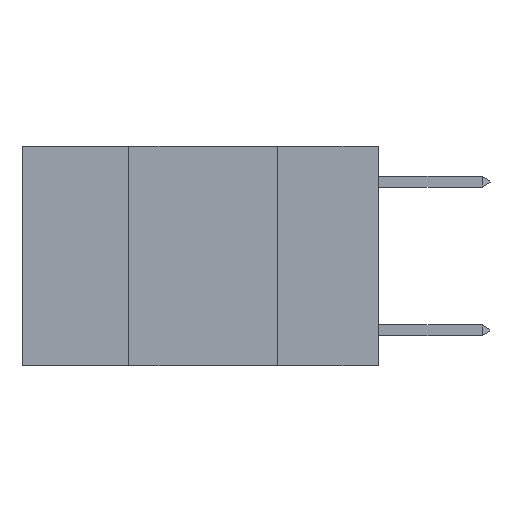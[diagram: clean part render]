
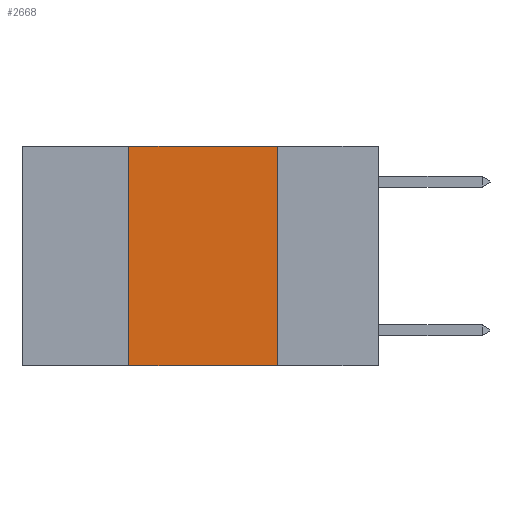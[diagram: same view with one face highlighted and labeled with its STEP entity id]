
A CAD part, left-side view. The second image highlights one B-rep face of the part: STEP entity #2668.
In plain terms, the highlighted planar face has unit normal (-1, 0, 0).
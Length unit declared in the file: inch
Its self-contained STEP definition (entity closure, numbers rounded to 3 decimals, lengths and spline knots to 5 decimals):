
#463 = EDGE_CURVE ( 'NONE', #13449, #3422, #1289, .T. ) ;
#912 = FACE_OUTER_BOUND ( 'NONE', #4843, .T. ) ;
#996 = DIRECTION ( 'NONE',  ( 0., 0., -1. ) ) ;
#1289 = LINE ( 'NONE', #12837, #10426 ) ;
#1579 = LINE ( 'NONE', #11140, #13060 ) ;
#1795 = EDGE_CURVE ( 'NONE', #3422, #13500, #10552, .T. ) ;
#1964 = CARTESIAN_POINT ( 'NONE',  ( 0., 0.17, 0. ) ) ;
#2070 = DIRECTION ( 'NONE',  ( 1., 0., 0. ) ) ;
#2234 = LINE ( 'NONE', #8668, #9821 ) ;
#2668 = ADVANCED_FACE ( 'NONE', ( #912 ), #3037, .F. ) ;
#2966 = VERTEX_POINT ( 'NONE', #6016 ) ;
#3037 = PLANE ( 'NONE',  #10551 ) ;
#3416 = DIRECTION ( 'NONE',  ( 0., -1., 0. ) ) ;
#3422 = VERTEX_POINT ( 'NONE', #1964 ) ;
#4843 = EDGE_LOOP ( 'NONE', ( #12612, #12504, #5500, #10301 ) ) ;
#5500 = ORIENTED_EDGE ( 'NONE', *, *, #12411, .F. ) ;
#6016 = CARTESIAN_POINT ( 'NONE',  ( 0., 0.42, -0.37 ) ) ;
#7295 = CARTESIAN_POINT ( 'NONE',  ( 0., 0.6, 0. ) ) ;
#7391 = CARTESIAN_POINT ( 'NONE',  ( 0., 0.17, 0. ) ) ;
#7983 = EDGE_CURVE ( 'NONE', #2966, #13500, #1579, .T. ) ;
#8668 = CARTESIAN_POINT ( 'NONE',  ( 0., 0.42, 0. ) ) ;
#9041 = CARTESIAN_POINT ( 'NONE',  ( 0., 0.42, 0. ) ) ;
#9384 = DIRECTION ( 'NONE',  ( 0., 0., -1. ) ) ;
#9821 = VECTOR ( 'NONE', #12889, 39.37008 ) ;
#10301 = ORIENTED_EDGE ( 'NONE', *, *, #7983, .T. ) ;
#10426 = VECTOR ( 'NONE', #3416, 39.37008 ) ;
#10551 = AXIS2_PLACEMENT_3D ( 'NONE', #7295, #2070, #9384 ) ;
#10552 = LINE ( 'NONE', #7391, #13448 ) ;
#10933 = DIRECTION ( 'NONE',  ( 0., -1., 0. ) ) ;
#11076 = CARTESIAN_POINT ( 'NONE',  ( 0., 0.17, -0.37 ) ) ;
#11140 = CARTESIAN_POINT ( 'NONE',  ( 0., 0.6, -0.37 ) ) ;
#12411 = EDGE_CURVE ( 'NONE', #2966, #13449, #2234, .T. ) ;
#12504 = ORIENTED_EDGE ( 'NONE', *, *, #463, .F. ) ;
#12612 = ORIENTED_EDGE ( 'NONE', *, *, #1795, .F. ) ;
#12837 = CARTESIAN_POINT ( 'NONE',  ( 0., 0.6, 0. ) ) ;
#12889 = DIRECTION ( 'NONE',  ( 0., 0., 1. ) ) ;
#13060 = VECTOR ( 'NONE', #10933, 39.37008 ) ;
#13448 = VECTOR ( 'NONE', #996, 39.37008 ) ;
#13449 = VERTEX_POINT ( 'NONE', #9041 ) ;
#13500 = VERTEX_POINT ( 'NONE', #11076 ) ;
